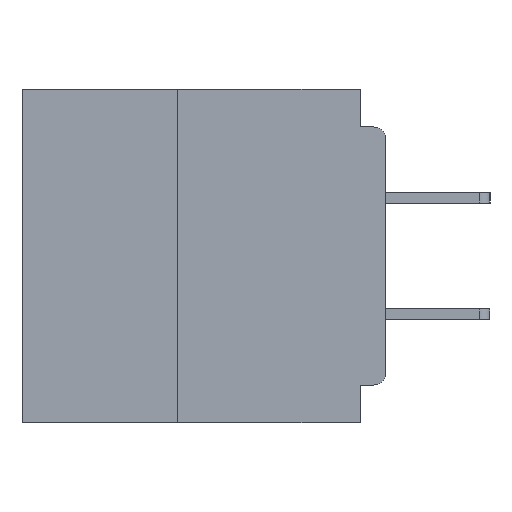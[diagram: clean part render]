
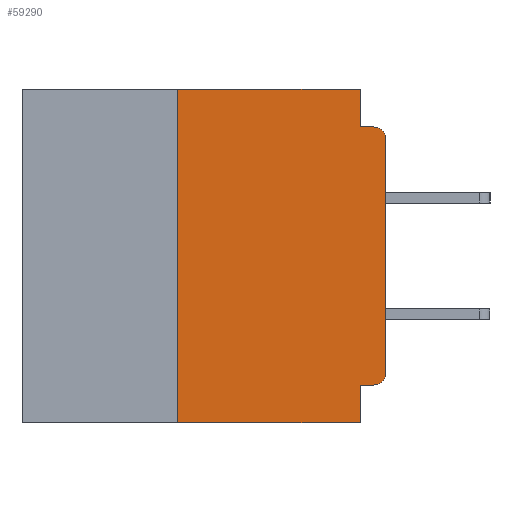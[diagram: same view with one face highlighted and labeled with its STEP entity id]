
A CAD part, left-side view. The second image highlights one B-rep face of the part: STEP entity #59290.
In plain terms, the highlighted planar face has unit normal (-1, 0, 0).
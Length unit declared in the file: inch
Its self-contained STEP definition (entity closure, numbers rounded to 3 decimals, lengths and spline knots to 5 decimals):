
#60 = VECTOR ( 'NONE', #5912, 39.37008 ) ;
#181 = CARTESIAN_POINT ( 'NONE',  ( 0., 0.015, -0.06 ) ) ;
#1549 = VERTEX_POINT ( 'NONE', #57996 ) ;
#2401 = EDGE_CURVE ( 'NONE', #23581, #32021, #6688, .T. ) ;
#5073 = DIRECTION ( 'NONE',  ( 0., 0., -1. ) ) ;
#5155 = VERTEX_POINT ( 'NONE', #19402 ) ;
#5912 = DIRECTION ( 'NONE',  ( 0., -1., 0. ) ) ;
#5984 = CIRCLE ( 'NONE', #61692, 0.015 ) ;
#6050 = CARTESIAN_POINT ( 'NONE',  ( 0., 0., -0.34 ) ) ;
#6289 = PLANE ( 'NONE',  #50672 ) ;
#6688 = LINE ( 'NONE', #26189, #56655 ) ;
#6825 = ORIENTED_EDGE ( 'NONE', *, *, #34050, .F. ) ;
#7363 = LINE ( 'NONE', #43898, #21797 ) ;
#7903 = CIRCLE ( 'NONE', #57985, 0.015 ) ;
#9974 = CARTESIAN_POINT ( 'NONE',  ( 0., 0.015, -0.34 ) ) ;
#10693 = CARTESIAN_POINT ( 'NONE',  ( 0., 0.031, -0.4 ) ) ;
#11146 = DIRECTION ( 'NONE',  ( 1., 0., 0. ) ) ;
#11440 = LINE ( 'NONE', #44885, #60 ) ;
#12583 = VERTEX_POINT ( 'NONE', #33462 ) ;
#12628 = ORIENTED_EDGE ( 'NONE', *, *, #43427, .T. ) ;
#12868 = EDGE_LOOP ( 'NONE', ( #12628, #30377, #62698, #45168, #13793, #48534, #15736, #51675, #6825, #49794 ) ) ;
#13511 = CARTESIAN_POINT ( 'NONE',  ( 0., 0.031, 0. ) ) ;
#13793 = ORIENTED_EDGE ( 'NONE', *, *, #52183, .F. ) ;
#14020 = VECTOR ( 'NONE', #46788, 39.37008 ) ;
#14939 = DIRECTION ( 'NONE',  ( 0., 0., -1. ) ) ;
#15475 = CARTESIAN_POINT ( 'NONE',  ( 0., 0.031, -0.355 ) ) ;
#15736 = ORIENTED_EDGE ( 'NONE', *, *, #2401, .T. ) ;
#16810 = VECTOR ( 'NONE', #24712, 39.37008 ) ;
#17399 = CARTESIAN_POINT ( 'NONE',  ( 0., 0.25, -0.4 ) ) ;
#19402 = CARTESIAN_POINT ( 'NONE',  ( 0., 0., -0.06 ) ) ;
#19695 = EDGE_CURVE ( 'NONE', #23581, #60440, #21227, .T. ) ;
#19830 = CARTESIAN_POINT ( 'NONE',  ( 0., 0., -0.355 ) ) ;
#20497 = DIRECTION ( 'NONE',  ( 0., 0., 1. ) ) ;
#21227 = LINE ( 'NONE', #27861, #45438 ) ;
#21797 = VECTOR ( 'NONE', #48737, 39.37008 ) ;
#23581 = VERTEX_POINT ( 'NONE', #17399 ) ;
#23977 = VERTEX_POINT ( 'NONE', #15475 ) ;
#24712 = DIRECTION ( 'NONE',  ( 0., 1., 0. ) ) ;
#24770 = EDGE_CURVE ( 'NONE', #12583, #25176, #11440, .T. ) ;
#24774 = CARTESIAN_POINT ( 'NONE',  ( 0., 0.015, -0.045 ) ) ;
#25176 = VERTEX_POINT ( 'NONE', #24774 ) ;
#26189 = CARTESIAN_POINT ( 'NONE',  ( 0., 0.437, -0.4 ) ) ;
#26900 = LINE ( 'NONE', #41963, #14020 ) ;
#27843 = EDGE_CURVE ( 'NONE', #1549, #12583, #48089, .T. ) ;
#27861 = CARTESIAN_POINT ( 'NONE',  ( 0., 0.25, -0.4 ) ) ;
#28076 = DIRECTION ( 'NONE',  ( 0., 0., 1. ) ) ;
#29180 = VECTOR ( 'NONE', #47334, 39.37008 ) ;
#30377 = ORIENTED_EDGE ( 'NONE', *, *, #45423, .T. ) ;
#32021 = VERTEX_POINT ( 'NONE', #10693 ) ;
#33462 = CARTESIAN_POINT ( 'NONE',  ( 0., 0.031, -0.045 ) ) ;
#34050 = EDGE_CURVE ( 'NONE', #35359, #23977, #55394, .T. ) ;
#34075 = DIRECTION ( 'NONE',  ( -1., 0., 0. ) ) ;
#35287 = CARTESIAN_POINT ( 'NONE',  ( 0., 0.437, 0. ) ) ;
#35359 = VERTEX_POINT ( 'NONE', #58591 ) ;
#36766 = LINE ( 'NONE', #49464, #49673 ) ;
#41963 = CARTESIAN_POINT ( 'NONE',  ( 0., 0.437, 0. ) ) ;
#43427 = EDGE_CURVE ( 'NONE', #43488, #5155, #36766, .T. ) ;
#43488 = VERTEX_POINT ( 'NONE', #6050 ) ;
#43898 = CARTESIAN_POINT ( 'NONE',  ( 0., 0.031, -0.4 ) ) ;
#43911 = DIRECTION ( 'NONE',  ( -1., 0., 0. ) ) ;
#43962 = EDGE_CURVE ( 'NONE', #35359, #43488, #7903, .T. ) ;
#44067 = CARTESIAN_POINT ( 'NONE',  ( 0., 0.25, 0. ) ) ;
#44885 = CARTESIAN_POINT ( 'NONE',  ( 0., 0., -0.045 ) ) ;
#45055 = DIRECTION ( 'NONE',  ( 0., 0., -1. ) ) ;
#45168 = ORIENTED_EDGE ( 'NONE', *, *, #27843, .F. ) ;
#45423 = EDGE_CURVE ( 'NONE', #5155, #25176, #5984, .T. ) ;
#45438 = VECTOR ( 'NONE', #28076, 39.37008 ) ;
#46788 = DIRECTION ( 'NONE',  ( 0., -1., 0. ) ) ;
#47334 = DIRECTION ( 'NONE',  ( 0., 0., -1. ) ) ;
#48089 = LINE ( 'NONE', #13511, #29180 ) ;
#48534 = ORIENTED_EDGE ( 'NONE', *, *, #19695, .F. ) ;
#48737 = DIRECTION ( 'NONE',  ( 0., 0., -1. ) ) ;
#49464 = CARTESIAN_POINT ( 'NONE',  ( 0., 0., 0. ) ) ;
#49673 = VECTOR ( 'NONE', #20497, 39.37008 ) ;
#49794 = ORIENTED_EDGE ( 'NONE', *, *, #43962, .T. ) ;
#49934 = FACE_OUTER_BOUND ( 'NONE', #12868, .T. ) ;
#50672 = AXIS2_PLACEMENT_3D ( 'NONE', #35287, #11146, #45055 ) ;
#51675 = ORIENTED_EDGE ( 'NONE', *, *, #56910, .F. ) ;
#52183 = EDGE_CURVE ( 'NONE', #60440, #1549, #26900, .T. ) ;
#55394 = LINE ( 'NONE', #19830, #16810 ) ;
#56655 = VECTOR ( 'NONE', #59996, 39.37008 ) ;
#56910 = EDGE_CURVE ( 'NONE', #23977, #32021, #7363, .T. ) ;
#57985 = AXIS2_PLACEMENT_3D ( 'NONE', #9974, #43911, #14939 ) ;
#57996 = CARTESIAN_POINT ( 'NONE',  ( 0., 0.031, 0. ) ) ;
#58591 = CARTESIAN_POINT ( 'NONE',  ( 0., 0.015, -0.355 ) ) ;
#59290 = ADVANCED_FACE ( 'NONE', ( #49934 ), #6289, .F. ) ;
#59996 = DIRECTION ( 'NONE',  ( 0., -1., 0. ) ) ;
#60440 = VERTEX_POINT ( 'NONE', #44067 ) ;
#61692 = AXIS2_PLACEMENT_3D ( 'NONE', #181, #34075, #5073 ) ;
#62698 = ORIENTED_EDGE ( 'NONE', *, *, #24770, .F. ) ;
